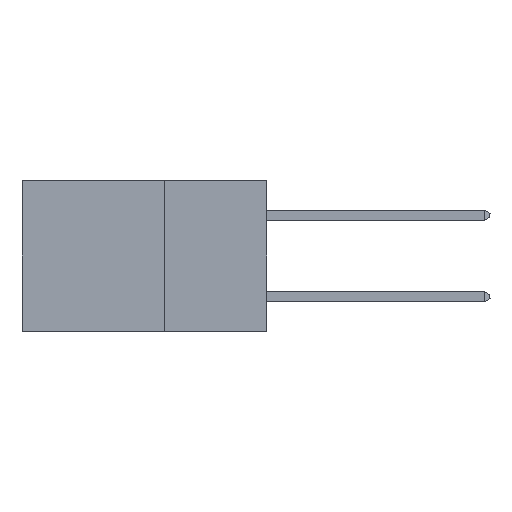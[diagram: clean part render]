
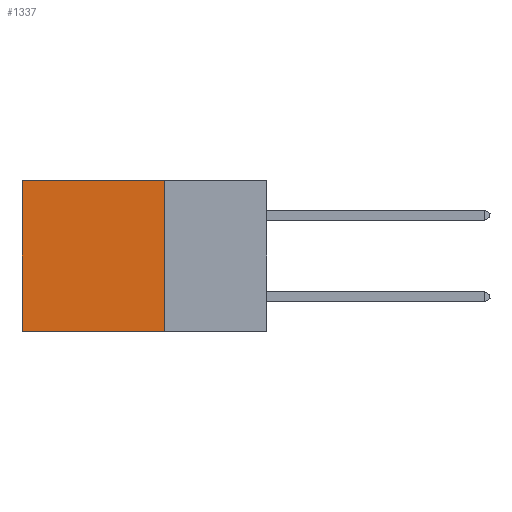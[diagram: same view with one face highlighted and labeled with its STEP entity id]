
A CAD part, left-side view. The second image highlights one B-rep face of the part: STEP entity #1337.
In plain terms, the highlighted planar face has unit normal (-1, 0, 0).
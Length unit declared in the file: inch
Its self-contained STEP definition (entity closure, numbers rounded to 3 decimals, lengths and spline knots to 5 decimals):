
#408 = LINE ( 'NONE', #15167, #32098 ) ;
#1337 = ADVANCED_FACE ( 'NONE', ( #6663 ), #11288, .F. ) ;
#2003 = VERTEX_POINT ( 'NONE', #11009 ) ;
#2876 = CARTESIAN_POINT ( 'NONE',  ( 0.2875, 0.6, 0. ) ) ;
#4087 = VECTOR ( 'NONE', #18186, 39.37008 ) ;
#4489 = LINE ( 'NONE', #10531, #4087 ) ;
#6660 = VERTEX_POINT ( 'NONE', #2876 ) ;
#6663 = FACE_OUTER_BOUND ( 'NONE', #19605, .T. ) ;
#7310 = ORIENTED_EDGE ( 'NONE', *, *, #23177, .F. ) ;
#8379 = ORIENTED_EDGE ( 'NONE', *, *, #11731, .T. ) ;
#10531 = CARTESIAN_POINT ( 'NONE',  ( 0.2875, 0.25, 0. ) ) ;
#11009 = CARTESIAN_POINT ( 'NONE',  ( 0.2875, 0.25, -0.37 ) ) ;
#11288 = PLANE ( 'NONE',  #14050 ) ;
#11731 = EDGE_CURVE ( 'NONE', #22812, #6660, #31143, .T. ) ;
#12301 = ORIENTED_EDGE ( 'NONE', *, *, #25025, .F. ) ;
#14050 = AXIS2_PLACEMENT_3D ( 'NONE', #31722, #23976, #16224 ) ;
#15167 = CARTESIAN_POINT ( 'NONE',  ( 0.2875, 0.6, 0. ) ) ;
#15970 = CARTESIAN_POINT ( 'NONE',  ( 0.2875, 0.6, -0.37 ) ) ;
#16126 = DIRECTION ( 'NONE',  ( 0., 1., 0. ) ) ;
#16224 = DIRECTION ( 'NONE',  ( 0., 0., -1. ) ) ;
#16362 = CARTESIAN_POINT ( 'NONE',  ( 0.2875, 0.25, 0. ) ) ;
#16427 = ORIENTED_EDGE ( 'NONE', *, *, #25342, .T. ) ;
#18186 = DIRECTION ( 'NONE',  ( 0., 0., -1. ) ) ;
#18942 = VECTOR ( 'NONE', #16126, 39.37008 ) ;
#19318 = DIRECTION ( 'NONE',  ( 0., 1., 0. ) ) ;
#19605 = EDGE_LOOP ( 'NONE', ( #16427, #7310, #12301, #8379 ) ) ;
#19775 = LINE ( 'NONE', #31623, #18942 ) ;
#19909 = CARTESIAN_POINT ( 'NONE',  ( 0.2875, 0.25, 0. ) ) ;
#22812 = VERTEX_POINT ( 'NONE', #19909 ) ;
#23177 = EDGE_CURVE ( 'NONE', #2003, #31082, #19775, .T. ) ;
#23976 = DIRECTION ( 'NONE',  ( 1., 0., 0. ) ) ;
#25025 = EDGE_CURVE ( 'NONE', #22812, #2003, #4489, .T. ) ;
#25342 = EDGE_CURVE ( 'NONE', #6660, #31082, #408, .T. ) ;
#25554 = VECTOR ( 'NONE', #19318, 39.37008 ) ;
#27992 = DIRECTION ( 'NONE',  ( 0., 0., -1. ) ) ;
#31082 = VERTEX_POINT ( 'NONE', #15970 ) ;
#31143 = LINE ( 'NONE', #16362, #25554 ) ;
#31623 = CARTESIAN_POINT ( 'NONE',  ( 0.2875, 0.25, -0.37 ) ) ;
#31722 = CARTESIAN_POINT ( 'NONE',  ( 0.2875, 0.25, 0. ) ) ;
#32098 = VECTOR ( 'NONE', #27992, 39.37008 ) ;
